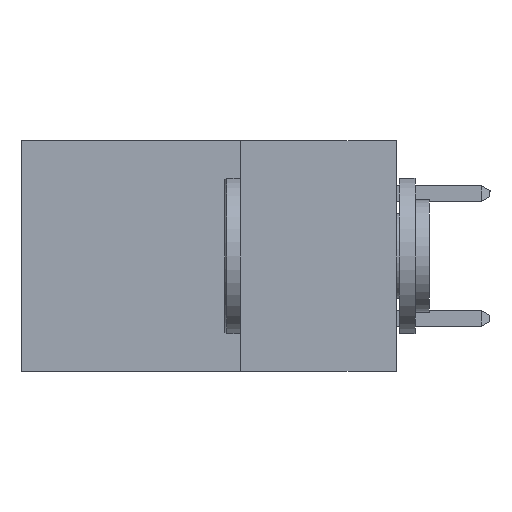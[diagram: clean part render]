
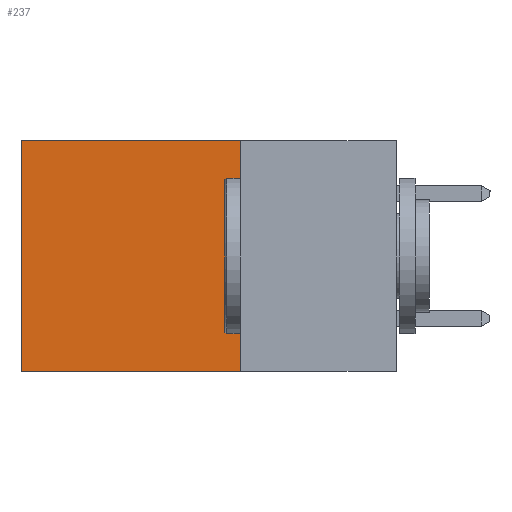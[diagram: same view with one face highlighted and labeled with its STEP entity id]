
A CAD part, left-side view. The second image highlights one B-rep face of the part: STEP entity #237.
In plain terms, the highlighted planar face has unit normal (-1, 0, 0).
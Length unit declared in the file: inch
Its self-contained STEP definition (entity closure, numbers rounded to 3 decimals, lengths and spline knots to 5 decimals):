
#237 = ADVANCED_FACE ( 'NONE', ( #1496 ), #5013, .F. ) ;
#1260 = VECTOR ( 'NONE', #7470, 39.37008 ) ;
#1436 = EDGE_CURVE ( 'NONE', #14468, #2956, #7926, .T. ) ;
#1496 = FACE_OUTER_BOUND ( 'NONE', #3673, .T. ) ;
#1829 = ORIENTED_EDGE ( 'NONE', *, *, #11111, .F. ) ;
#2364 = CARTESIAN_POINT ( 'NONE',  ( 0.2615, 0.25, -0.37 ) ) ;
#2542 = ORIENTED_EDGE ( 'NONE', *, *, #5174, .F. ) ;
#2728 = CARTESIAN_POINT ( 'NONE',  ( 0.2615, 0.25, -0.37 ) ) ;
#2763 = ORIENTED_EDGE ( 'NONE', *, *, #1436, .T. ) ;
#2956 = VERTEX_POINT ( 'NONE', #4353 ) ;
#3107 = CARTESIAN_POINT ( 'NONE',  ( 0.2615, 0.25, 0. ) ) ;
#3673 = EDGE_LOOP ( 'NONE', ( #11712, #1829, #2542, #2763 ) ) ;
#3803 = VERTEX_POINT ( 'NONE', #11589 ) ;
#3998 = LINE ( 'NONE', #9650, #7484 ) ;
#4241 = DIRECTION ( 'NONE',  ( 0., 0., -1. ) ) ;
#4353 = CARTESIAN_POINT ( 'NONE',  ( 0.2615, 0.6, 0. ) ) ;
#5013 = PLANE ( 'NONE',  #10028 ) ;
#5174 = EDGE_CURVE ( 'NONE', #14468, #14113, #6660, .T. ) ;
#5304 = DIRECTION ( 'NONE',  ( 0., 0., -1. ) ) ;
#5892 = CARTESIAN_POINT ( 'NONE',  ( 0.2615, 0.25, -0.37 ) ) ;
#6660 = LINE ( 'NONE', #15111, #6881 ) ;
#6881 = VECTOR ( 'NONE', #4241, 39.37008 ) ;
#7090 = DIRECTION ( 'NONE',  ( 1., 0., 0. ) ) ;
#7470 = DIRECTION ( 'NONE',  ( 0., 1., 0. ) ) ;
#7484 = VECTOR ( 'NONE', #5304, 39.37008 ) ;
#7926 = LINE ( 'NONE', #3107, #12441 ) ;
#9650 = CARTESIAN_POINT ( 'NONE',  ( 0.2615, 0.6, -0.37 ) ) ;
#9916 = CARTESIAN_POINT ( 'NONE',  ( 0.2615, 0.25, 0. ) ) ;
#10028 = AXIS2_PLACEMENT_3D ( 'NONE', #2364, #7090, #11060 ) ;
#11060 = DIRECTION ( 'NONE',  ( 0., 0., -1. ) ) ;
#11111 = EDGE_CURVE ( 'NONE', #14113, #3803, #14347, .T. ) ;
#11589 = CARTESIAN_POINT ( 'NONE',  ( 0.2615, 0.6, -0.37 ) ) ;
#11712 = ORIENTED_EDGE ( 'NONE', *, *, #15325, .T. ) ;
#12441 = VECTOR ( 'NONE', #13950, 39.37008 ) ;
#13950 = DIRECTION ( 'NONE',  ( 0., 1., 0. ) ) ;
#14113 = VERTEX_POINT ( 'NONE', #5892 ) ;
#14347 = LINE ( 'NONE', #2728, #1260 ) ;
#14468 = VERTEX_POINT ( 'NONE', #9916 ) ;
#15111 = CARTESIAN_POINT ( 'NONE',  ( 0.2615, 0.25, -0.37 ) ) ;
#15325 = EDGE_CURVE ( 'NONE', #2956, #3803, #3998, .T. ) ;
